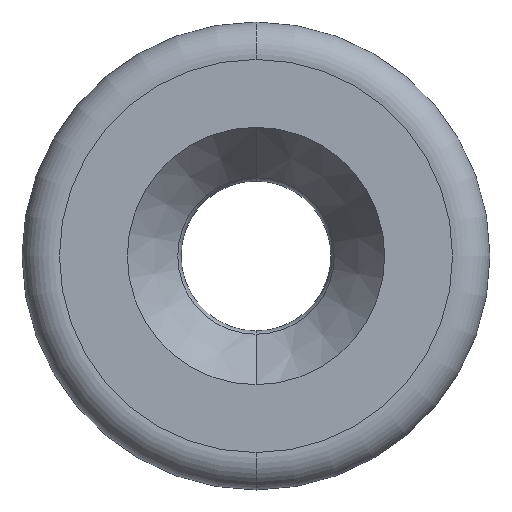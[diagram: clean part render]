
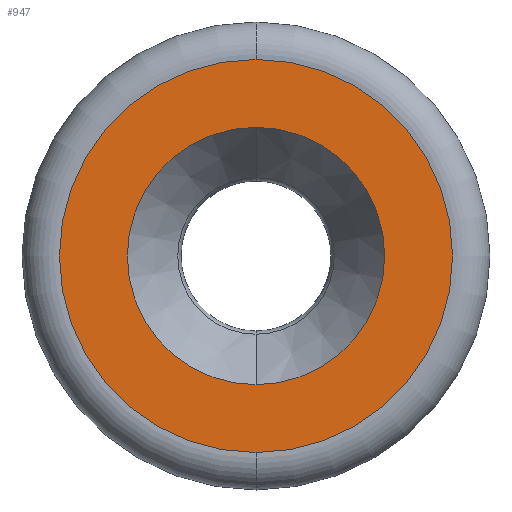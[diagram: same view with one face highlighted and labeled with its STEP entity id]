
A CAD part, front view. The second image highlights one B-rep face of the part: STEP entity #947.
In plain terms, the highlighted planar face has unit normal (0, -1, 0).
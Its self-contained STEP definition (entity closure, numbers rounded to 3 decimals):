
#6 = CIRCLE ( 'NONE', #1251, 1.375 ) ;
#84 = VERTEX_POINT ( 'NONE', #872 ) ;
#123 = DIRECTION ( 'NONE',  ( 0., -1., 0. ) ) ;
#200 = EDGE_LOOP ( 'NONE', ( #1624, #691 ) ) ;
#246 = CIRCLE ( 'NONE', #481, 2.1 ) ;
#247 = AXIS2_PLACEMENT_3D ( 'NONE', #710, #682, #1191 ) ;
#306 = CARTESIAN_POINT ( 'NONE',  ( 0., -11.05, -1.15 ) ) ;
#323 = CARTESIAN_POINT ( 'NONE',  ( 0., -11.05, -1.15 ) ) ;
#425 = PLANE ( 'NONE',  #1340 ) ;
#450 = EDGE_CURVE ( 'NONE', #967, #84, #6, .T. ) ;
#481 = AXIS2_PLACEMENT_3D ( 'NONE', #726, #123, #742 ) ;
#550 = FACE_OUTER_BOUND ( 'NONE', #200, .T. ) ;
#557 = AXIS2_PLACEMENT_3D ( 'NONE', #1230, #873, #1385 ) ;
#571 = CARTESIAN_POINT ( 'NONE',  ( 0., -11.05, 0.95 ) ) ;
#573 = EDGE_CURVE ( 'NONE', #963, #1322, #246, .T. ) ;
#682 = DIRECTION ( 'NONE',  ( 0., 1., 0. ) ) ;
#691 = ORIENTED_EDGE ( 'NONE', *, *, #573, .T. ) ;
#710 = CARTESIAN_POINT ( 'NONE',  ( 0., -11.05, -1.15 ) ) ;
#726 = CARTESIAN_POINT ( 'NONE',  ( 0., -11.05, -1.15 ) ) ;
#742 = DIRECTION ( 'NONE',  ( 0., 0., -1. ) ) ;
#827 = DIRECTION ( 'NONE',  ( 0., -1., 0. ) ) ;
#872 = CARTESIAN_POINT ( 'NONE',  ( 0., -11.05, 0.225 ) ) ;
#873 = DIRECTION ( 'NONE',  ( 0., 1., 0. ) ) ;
#923 = CIRCLE ( 'NONE', #247, 1.375 ) ;
#938 = FACE_BOUND ( 'NONE', #1449, .T. ) ;
#947 = ADVANCED_FACE ( 'NONE', ( #938, #550 ), #425, .T. ) ;
#963 = VERTEX_POINT ( 'NONE', #1470 ) ;
#964 = CARTESIAN_POINT ( 'NONE',  ( 0., -11.05, -2.525 ) ) ;
#967 = VERTEX_POINT ( 'NONE', #964 ) ;
#1155 = ORIENTED_EDGE ( 'NONE', *, *, #1311, .T. ) ;
#1191 = DIRECTION ( 'NONE',  ( 0., 0., -1. ) ) ;
#1199 = DIRECTION ( 'NONE',  ( 0., 0., -1. ) ) ;
#1219 = ORIENTED_EDGE ( 'NONE', *, *, #450, .F. ) ;
#1230 = CARTESIAN_POINT ( 'NONE',  ( 0., -11.05, -1.15 ) ) ;
#1251 = AXIS2_PLACEMENT_3D ( 'NONE', #323, #827, #1335 ) ;
#1276 = CIRCLE ( 'NONE', #557, 2.1 ) ;
#1311 = EDGE_CURVE ( 'NONE', #967, #84, #923, .T. ) ;
#1322 = VERTEX_POINT ( 'NONE', #571 ) ;
#1335 = DIRECTION ( 'NONE',  ( 0., 0., -1. ) ) ;
#1340 = AXIS2_PLACEMENT_3D ( 'NONE', #306, #1565, #1199 ) ;
#1385 = DIRECTION ( 'NONE',  ( 0., 0., -1. ) ) ;
#1410 = EDGE_CURVE ( 'NONE', #963, #1322, #1276, .T. ) ;
#1449 = EDGE_LOOP ( 'NONE', ( #1219, #1155 ) ) ;
#1470 = CARTESIAN_POINT ( 'NONE',  ( 0., -11.05, -3.25 ) ) ;
#1565 = DIRECTION ( 'NONE',  ( 0., -1., 0. ) ) ;
#1624 = ORIENTED_EDGE ( 'NONE', *, *, #1410, .F. ) ;
